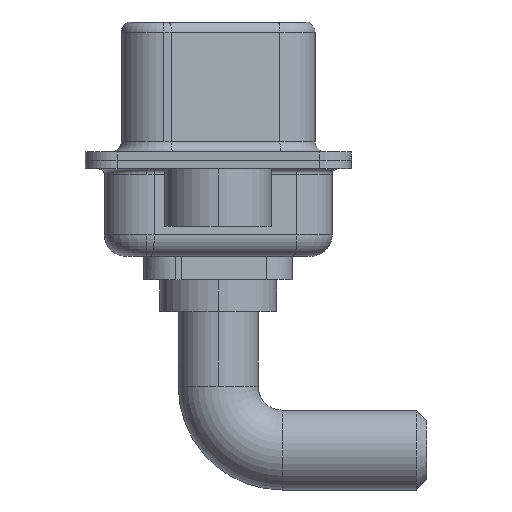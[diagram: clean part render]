
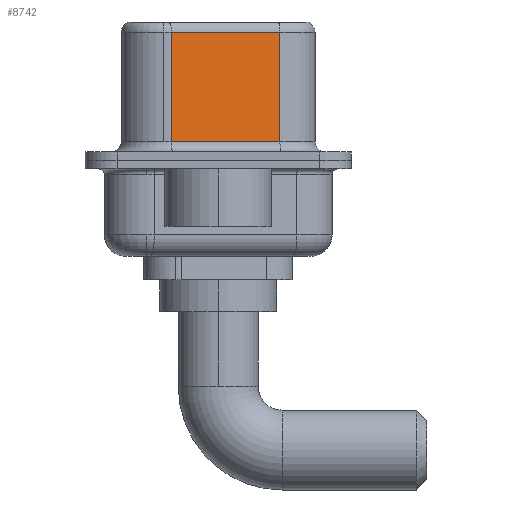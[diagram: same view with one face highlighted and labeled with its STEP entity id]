
A CAD part, left-side view. The second image highlights one B-rep face of the part: STEP entity #8742.
In plain terms, the highlighted planar face has unit normal (-0.985, -0.174, 0).
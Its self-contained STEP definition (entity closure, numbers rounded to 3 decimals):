
#156 = EDGE_CURVE ( 'NONE', #6773, #387, #1098, .T. ) ;
#387 = VERTEX_POINT ( 'NONE', #12844 ) ;
#1098 = LINE ( 'NONE', #11329, #6397 ) ;
#1390 = ORIENTED_EDGE ( 'NONE', *, *, #13614, .T. ) ;
#1720 = DIRECTION ( 'NONE',  ( -0.174, 0.985, 0. ) ) ;
#2857 = ORIENTED_EDGE ( 'NONE', *, *, #5269, .F. ) ;
#2950 = DIRECTION ( 'NONE',  ( 0.985, 0.174, 0. ) ) ;
#3197 = CARTESIAN_POINT ( 'NONE',  ( 4.58, -2.897, 0.9 ) ) ;
#3259 = LINE ( 'NONE', #7725, #3697 ) ;
#3389 = ORIENTED_EDGE ( 'NONE', *, *, #156, .T. ) ;
#3530 = CARTESIAN_POINT ( 'NONE',  ( 4.58, -2.897, 6.02 ) ) ;
#3697 = VECTOR ( 'NONE', #5506, 1000. ) ;
#3855 = LINE ( 'NONE', #3998, #14408 ) ;
#3998 = CARTESIAN_POINT ( 'NONE',  ( 4.58, -2.897, 0.9 ) ) ;
#5269 = EDGE_CURVE ( 'NONE', #6773, #13167, #6769, .T. ) ;
#5506 = DIRECTION ( 'NONE',  ( 0., 0., -1. ) ) ;
#6397 = VECTOR ( 'NONE', #10010, 1000. ) ;
#6769 = LINE ( 'NONE', #9207, #14272 ) ;
#6773 = VERTEX_POINT ( 'NONE', #3530 ) ;
#7725 = CARTESIAN_POINT ( 'NONE',  ( 3.68, 2.203, 6.52 ) ) ;
#8469 = DIRECTION ( 'NONE',  ( 0.174, -0.985, 0. ) ) ;
#8742 = ADVANCED_FACE ( 'NONE', ( #11735 ), #14197, .F. ) ;
#8956 = CARTESIAN_POINT ( 'NONE',  ( 3.68, 2.203, 0.9 ) ) ;
#9207 = CARTESIAN_POINT ( 'NONE',  ( 4.58, -2.897, 6.52 ) ) ;
#9880 = EDGE_LOOP ( 'NONE', ( #2857, #3389, #1390, #13985 ) ) ;
#10010 = DIRECTION ( 'NONE',  ( -0.174, 0.985, 0. ) ) ;
#11131 = AXIS2_PLACEMENT_3D ( 'NONE', #13917, #2950, #1720 ) ;
#11223 = DIRECTION ( 'NONE',  ( 0., 0., -1. ) ) ;
#11329 = CARTESIAN_POINT ( 'NONE',  ( 4.58, -2.897, 6.02 ) ) ;
#11735 = FACE_OUTER_BOUND ( 'NONE', #9880, .T. ) ;
#12122 = VERTEX_POINT ( 'NONE', #8956 ) ;
#12844 = CARTESIAN_POINT ( 'NONE',  ( 3.68, 2.203, 6.02 ) ) ;
#13167 = VERTEX_POINT ( 'NONE', #3197 ) ;
#13594 = EDGE_CURVE ( 'NONE', #12122, #13167, #3855, .T. ) ;
#13614 = EDGE_CURVE ( 'NONE', #387, #12122, #3259, .T. ) ;
#13917 = CARTESIAN_POINT ( 'NONE',  ( 4.58, -2.897, 6.52 ) ) ;
#13985 = ORIENTED_EDGE ( 'NONE', *, *, #13594, .T. ) ;
#14197 = PLANE ( 'NONE',  #11131 ) ;
#14272 = VECTOR ( 'NONE', #11223, 1000. ) ;
#14408 = VECTOR ( 'NONE', #8469, 1000. ) ;
